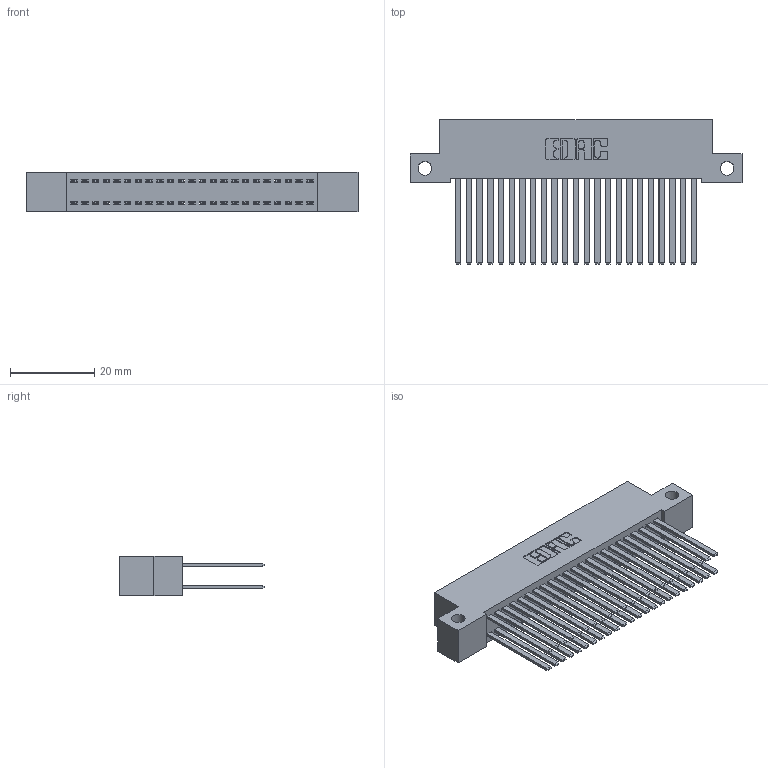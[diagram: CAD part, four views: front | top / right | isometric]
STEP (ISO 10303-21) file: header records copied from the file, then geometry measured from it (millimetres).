
FILE_DESCRIPTION (( 'STEP AP203' ), '1' );
FILE_NAME ('342-046-544-212.STEP', '2018-08-12T16:29:24', ( '' ), ( '' ), 'SwSTEP 2.0', 'SolidWorks 2016', '' );
FILE_SCHEMA (( 'CONFIG_CONTROL_DESIGN' ));
Length unit declared in the file: inch
Products named in the file (3): 342 Part_Side Mount; 345-292-001_345-293-144; 342-046-544-212
Assembly tree (47 placements, depth 2):
  342-046-544-212
    342 Part_Side Mount
    345-292-001_345-293-144  x46
Bounding box: 78.74 x 34.3 x 9.4 mm (x, y, z)
Volume: 7555.7 mm3; surface area: 13456.7 mm2
Topology: 47 solids, 47 shells, 2226 faces, 6601 edges, 4338 vertices
Faces by surface type: plane 1538, cylinder 688
Entity records: 16941 total; most frequent: CARTESIAN_POINT 2826, ORIENTED_EDGE 2762, DIRECTION 2445, EDGE_CURVE 1381, LINE 1257, VECTOR 1257, VERTEX_POINT 918, AXIS2_PLACEMENT_3D 594
